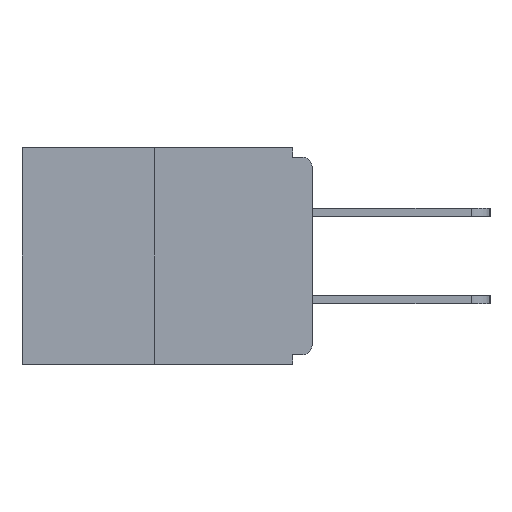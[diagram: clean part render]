
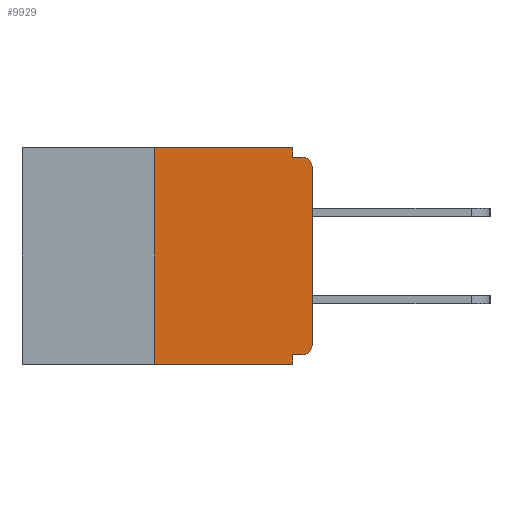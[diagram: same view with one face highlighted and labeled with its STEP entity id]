
A CAD part, left-side view. The second image highlights one B-rep face of the part: STEP entity #9929.
In plain terms, the highlighted planar face has unit normal (-1, 0, 0).
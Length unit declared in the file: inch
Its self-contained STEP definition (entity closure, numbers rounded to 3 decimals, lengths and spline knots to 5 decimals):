
#136 = DIRECTION ( 'NONE',  ( 0., 0., 1. ) ) ;
#692 = ORIENTED_EDGE ( 'NONE', *, *, #5319, .F. ) ;
#835 = VECTOR ( 'NONE', #3569, 39.37008 ) ;
#950 = VECTOR ( 'NONE', #9396, 39.37008 ) ;
#1414 = ORIENTED_EDGE ( 'NONE', *, *, #15892, .T. ) ;
#1927 = EDGE_CURVE ( 'NONE', #3759, #11160, #13708, .T. ) ;
#2256 = EDGE_LOOP ( 'NONE', ( #692, #11126, #14927, #11629, #10746, #1414, #6558, #12418, #17058, #14707 ) ) ;
#2434 = DIRECTION ( 'NONE',  ( 0., 0., -1. ) ) ;
#2441 = PLANE ( 'NONE',  #13675 ) ;
#2603 = VERTEX_POINT ( 'NONE', #7898 ) ;
#3242 = CARTESIAN_POINT ( 'NONE',  ( 0., 0.031, -0.328 ) ) ;
#3569 = DIRECTION ( 'NONE',  ( 0., 0., -1. ) ) ;
#3605 = CARTESIAN_POINT ( 'NONE',  ( 0., 0.46, 0. ) ) ;
#3653 = VECTOR ( 'NONE', #13239, 39.37008 ) ;
#3759 = VERTEX_POINT ( 'NONE', #5147 ) ;
#3949 = CARTESIAN_POINT ( 'NONE',  ( 0., 0.031, 0. ) ) ;
#4355 = VECTOR ( 'NONE', #136, 39.37008 ) ;
#4610 = AXIS2_PLACEMENT_3D ( 'NONE', #14548, #15717, #2434 ) ;
#4741 = LINE ( 'NONE', #14936, #13092 ) ;
#5047 = DIRECTION ( 'NONE',  ( 1., 0., 0. ) ) ;
#5147 = CARTESIAN_POINT ( 'NONE',  ( 0., 0.015, -0.328 ) ) ;
#5319 = EDGE_CURVE ( 'NONE', #12392, #13236, #16213, .T. ) ;
#5373 = DIRECTION ( 'NONE',  ( 0., -1., 0. ) ) ;
#5447 = CARTESIAN_POINT ( 'NONE',  ( 0., 0.25, 0. ) ) ;
#5497 = DIRECTION ( 'NONE',  ( 0., -1., 0. ) ) ;
#5615 = LINE ( 'NONE', #11511, #13861 ) ;
#6365 = CARTESIAN_POINT ( 'NONE',  ( 0., 0.015, -0.015 ) ) ;
#6558 = ORIENTED_EDGE ( 'NONE', *, *, #18122, .T. ) ;
#6630 = CARTESIAN_POINT ( 'NONE',  ( 0., 0.031, 0. ) ) ;
#6694 = VERTEX_POINT ( 'NONE', #12054 ) ;
#6847 = VERTEX_POINT ( 'NONE', #18858 ) ;
#6958 = CARTESIAN_POINT ( 'NONE',  ( 0., 0., -0.015 ) ) ;
#7362 = CARTESIAN_POINT ( 'NONE',  ( 0., 0.46, 0. ) ) ;
#7592 = EDGE_CURVE ( 'NONE', #11160, #2603, #5615, .T. ) ;
#7689 = CIRCLE ( 'NONE', #4610, 0.015 ) ;
#7765 = CARTESIAN_POINT ( 'NONE',  ( 0., 0., -0.03 ) ) ;
#7898 = CARTESIAN_POINT ( 'NONE',  ( 0., 0.031, -0.343 ) ) ;
#9263 = EDGE_CURVE ( 'NONE', #6694, #12392, #4741, .T. ) ;
#9362 = DIRECTION ( 'NONE',  ( -1., 0., 0. ) ) ;
#9396 = DIRECTION ( 'NONE',  ( 0., 1., 0. ) ) ;
#9929 = ADVANCED_FACE ( 'NONE', ( #15722 ), #2441, .F. ) ;
#10015 = LINE ( 'NONE', #15957, #11332 ) ;
#10073 = DIRECTION ( 'NONE',  ( 0., 0., -1. ) ) ;
#10168 = VERTEX_POINT ( 'NONE', #6365 ) ;
#10436 = AXIS2_PLACEMENT_3D ( 'NONE', #16744, #9362, #10795 ) ;
#10746 = ORIENTED_EDGE ( 'NONE', *, *, #1927, .F. ) ;
#10795 = DIRECTION ( 'NONE',  ( 0., 0., -1. ) ) ;
#11018 = DIRECTION ( 'NONE',  ( 0., 0., -1. ) ) ;
#11126 = ORIENTED_EDGE ( 'NONE', *, *, #9263, .F. ) ;
#11160 = VERTEX_POINT ( 'NONE', #3242 ) ;
#11332 = VECTOR ( 'NONE', #5373, 39.37008 ) ;
#11511 = CARTESIAN_POINT ( 'NONE',  ( 0., 0.031, -0.343 ) ) ;
#11629 = ORIENTED_EDGE ( 'NONE', *, *, #7592, .F. ) ;
#11813 = LINE ( 'NONE', #14587, #4355 ) ;
#11887 = EDGE_CURVE ( 'NONE', #13236, #6847, #16742, .T. ) ;
#12006 = EDGE_CURVE ( 'NONE', #6694, #2603, #10015, .T. ) ;
#12054 = CARTESIAN_POINT ( 'NONE',  ( 0., 0.25, -0.343 ) ) ;
#12392 = VERTEX_POINT ( 'NONE', #5447 ) ;
#12418 = ORIENTED_EDGE ( 'NONE', *, *, #15150, .T. ) ;
#12428 = CARTESIAN_POINT ( 'NONE',  ( 0., 0., -0.313 ) ) ;
#13092 = VECTOR ( 'NONE', #15137, 39.37008 ) ;
#13236 = VERTEX_POINT ( 'NONE', #3949 ) ;
#13239 = DIRECTION ( 'NONE',  ( 0., -1., 0. ) ) ;
#13675 = AXIS2_PLACEMENT_3D ( 'NONE', #3605, #5047, #11018 ) ;
#13708 = LINE ( 'NONE', #18137, #950 ) ;
#13861 = VECTOR ( 'NONE', #10073, 39.37008 ) ;
#14548 = CARTESIAN_POINT ( 'NONE',  ( 0., 0.015, -0.313 ) ) ;
#14587 = CARTESIAN_POINT ( 'NONE',  ( 0., 0., 0. ) ) ;
#14707 = ORIENTED_EDGE ( 'NONE', *, *, #11887, .F. ) ;
#14927 = ORIENTED_EDGE ( 'NONE', *, *, #12006, .T. ) ;
#14936 = CARTESIAN_POINT ( 'NONE',  ( 0., 0.25, 0. ) ) ;
#15137 = DIRECTION ( 'NONE',  ( 0., 0., 1. ) ) ;
#15150 = EDGE_CURVE ( 'NONE', #18331, #10168, #16254, .T. ) ;
#15218 = VERTEX_POINT ( 'NONE', #12428 ) ;
#15717 = DIRECTION ( 'NONE',  ( -1., 0., 0. ) ) ;
#15722 = FACE_OUTER_BOUND ( 'NONE', #2256, .T. ) ;
#15892 = EDGE_CURVE ( 'NONE', #3759, #15218, #7689, .T. ) ;
#15899 = EDGE_CURVE ( 'NONE', #6847, #10168, #18783, .T. ) ;
#15957 = CARTESIAN_POINT ( 'NONE',  ( 0., 0.46, -0.343 ) ) ;
#15979 = VECTOR ( 'NONE', #5497, 39.37008 ) ;
#16213 = LINE ( 'NONE', #7362, #3653 ) ;
#16254 = CIRCLE ( 'NONE', #10436, 0.015 ) ;
#16742 = LINE ( 'NONE', #6630, #835 ) ;
#16744 = CARTESIAN_POINT ( 'NONE',  ( 0., 0.015, -0.03 ) ) ;
#17058 = ORIENTED_EDGE ( 'NONE', *, *, #15899, .F. ) ;
#18122 = EDGE_CURVE ( 'NONE', #15218, #18331, #11813, .T. ) ;
#18137 = CARTESIAN_POINT ( 'NONE',  ( 0., 0., -0.328 ) ) ;
#18331 = VERTEX_POINT ( 'NONE', #7765 ) ;
#18783 = LINE ( 'NONE', #6958, #15979 ) ;
#18858 = CARTESIAN_POINT ( 'NONE',  ( 0., 0.031, -0.015 ) ) ;
